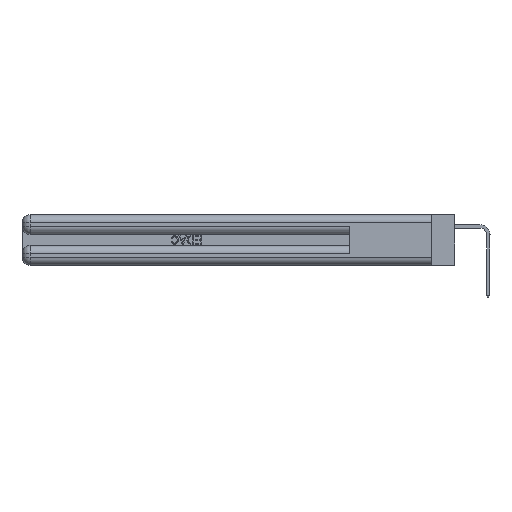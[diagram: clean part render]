
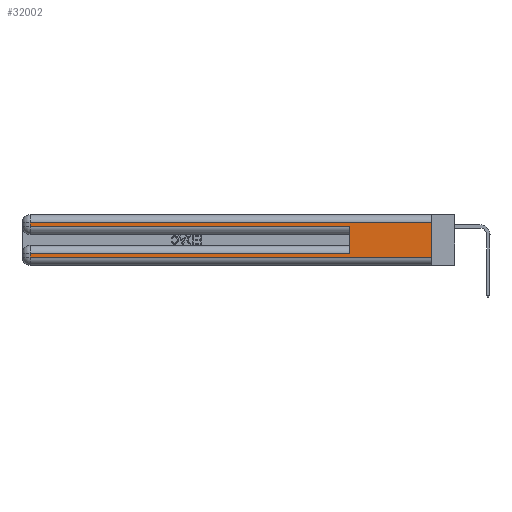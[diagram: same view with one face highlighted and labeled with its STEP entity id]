
A CAD part, left-side view. The second image highlights one B-rep face of the part: STEP entity #32002.
In plain terms, the highlighted planar face has unit normal (-1, 0, 0).
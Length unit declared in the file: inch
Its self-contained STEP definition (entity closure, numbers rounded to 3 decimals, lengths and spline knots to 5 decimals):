
#416 = CARTESIAN_POINT ( 'NONE',  ( 0., 2.94, 0.285 ) ) ;
#809 = VERTEX_POINT ( 'NONE', #416 ) ;
#941 = LINE ( 'NONE', #19264, #25725 ) ;
#985 = EDGE_CURVE ( 'NONE', #2743, #10307, #14815, .T. ) ;
#2058 = DIRECTION ( 'NONE',  ( 0., 0., -1. ) ) ;
#2743 = VERTEX_POINT ( 'NONE', #41487 ) ;
#3011 = VECTOR ( 'NONE', #13478, 39.37008 ) ;
#3036 = CARTESIAN_POINT ( 'NONE',  ( 0., 2.94, 0.31 ) ) ;
#3138 = DIRECTION ( 'NONE',  ( 0., 0., -1. ) ) ;
#3290 = FACE_OUTER_BOUND ( 'NONE', #34576, .T. ) ;
#3439 = CARTESIAN_POINT ( 'NONE',  ( 0., 0., 0.285 ) ) ;
#3688 = VERTEX_POINT ( 'NONE', #37135 ) ;
#4161 = VERTEX_POINT ( 'NONE', #39572 ) ;
#4561 = VERTEX_POINT ( 'NONE', #3036 ) ;
#6394 = DIRECTION ( 'NONE',  ( 0., 1., 0. ) ) ;
#6622 = LINE ( 'NONE', #3439, #31347 ) ;
#8910 = CARTESIAN_POINT ( 'NONE',  ( 0., 2.94, 0.37 ) ) ;
#9658 = LINE ( 'NONE', #32082, #36260 ) ;
#9823 = ORIENTED_EDGE ( 'NONE', *, *, #39728, .F. ) ;
#10307 = VERTEX_POINT ( 'NONE', #21825 ) ;
#10595 = VECTOR ( 'NONE', #39861, 39.37008 ) ;
#11454 = DIRECTION ( 'NONE',  ( 0., 0., 1. ) ) ;
#11680 = LINE ( 'NONE', #13610, #3011 ) ;
#13478 = DIRECTION ( 'NONE',  ( 0., -1., 0. ) ) ;
#13610 = CARTESIAN_POINT ( 'NONE',  ( 0., 0., 0.06 ) ) ;
#14056 = EDGE_CURVE ( 'NONE', #809, #10307, #6622, .T. ) ;
#14815 = LINE ( 'NONE', #27477, #23343 ) ;
#14848 = LINE ( 'NONE', #33110, #22363 ) ;
#14862 = EDGE_CURVE ( 'NONE', #4161, #3688, #11680, .T. ) ;
#16480 = ORIENTED_EDGE ( 'NONE', *, *, #25619, .T. ) ;
#17704 = CARTESIAN_POINT ( 'NONE',  ( 0., 0., 0.31 ) ) ;
#17847 = CARTESIAN_POINT ( 'NONE',  ( 0., 2.94, 0.085 ) ) ;
#19086 = LINE ( 'NONE', #8910, #35114 ) ;
#19155 = LINE ( 'NONE', #27089, #10595 ) ;
#19264 = CARTESIAN_POINT ( 'NONE',  ( 0., 2.94, 0.37 ) ) ;
#21438 = DIRECTION ( 'NONE',  ( 1., 0., 0. ) ) ;
#21825 = CARTESIAN_POINT ( 'NONE',  ( 0., 0.6, 0.285 ) ) ;
#22363 = VECTOR ( 'NONE', #26653, 39.37008 ) ;
#23233 = VERTEX_POINT ( 'NONE', #17847 ) ;
#23343 = VECTOR ( 'NONE', #11454, 39.37008 ) ;
#24822 = EDGE_CURVE ( 'NONE', #4561, #809, #941, .T. ) ;
#25619 = EDGE_CURVE ( 'NONE', #23233, #4161, #19086, .T. ) ;
#25725 = VECTOR ( 'NONE', #3138, 39.37008 ) ;
#26653 = DIRECTION ( 'NONE',  ( 0., 0., -1. ) ) ;
#26655 = AXIS2_PLACEMENT_3D ( 'NONE', #40238, #21438, #2058 ) ;
#27089 = CARTESIAN_POINT ( 'NONE',  ( 0., 0., 0.085 ) ) ;
#27477 = CARTESIAN_POINT ( 'NONE',  ( 0., 0.6, 0.145 ) ) ;
#29108 = EDGE_CURVE ( 'NONE', #41019, #4561, #9658, .T. ) ;
#29252 = DIRECTION ( 'NONE',  ( 0., -1., 0. ) ) ;
#29908 = EDGE_CURVE ( 'NONE', #2743, #23233, #19155, .T. ) ;
#31347 = VECTOR ( 'NONE', #29252, 39.37008 ) ;
#31430 = DIRECTION ( 'NONE',  ( 0., 0., -1. ) ) ;
#31756 = ORIENTED_EDGE ( 'NONE', *, *, #14056, .T. ) ;
#32002 = ADVANCED_FACE ( 'NONE', ( #3290 ), #40512, .F. ) ;
#32082 = CARTESIAN_POINT ( 'NONE',  ( 0., 0., 0.31 ) ) ;
#32940 = ORIENTED_EDGE ( 'NONE', *, *, #985, .F. ) ;
#33110 = CARTESIAN_POINT ( 'NONE',  ( 0., 0., 0.37 ) ) ;
#34576 = EDGE_LOOP ( 'NONE', ( #9823, #37883, #37714, #31756, #32940, #37865, #16480, #35049 ) ) ;
#35049 = ORIENTED_EDGE ( 'NONE', *, *, #14862, .T. ) ;
#35114 = VECTOR ( 'NONE', #31430, 39.37008 ) ;
#36260 = VECTOR ( 'NONE', #6394, 39.37008 ) ;
#37135 = CARTESIAN_POINT ( 'NONE',  ( 0., 0., 0.06 ) ) ;
#37714 = ORIENTED_EDGE ( 'NONE', *, *, #24822, .T. ) ;
#37865 = ORIENTED_EDGE ( 'NONE', *, *, #29908, .T. ) ;
#37883 = ORIENTED_EDGE ( 'NONE', *, *, #29108, .T. ) ;
#39572 = CARTESIAN_POINT ( 'NONE',  ( 0., 2.94, 0.06 ) ) ;
#39728 = EDGE_CURVE ( 'NONE', #41019, #3688, #14848, .T. ) ;
#39861 = DIRECTION ( 'NONE',  ( 0., 1., 0. ) ) ;
#40238 = CARTESIAN_POINT ( 'NONE',  ( 0., 0., 0.37 ) ) ;
#40512 = PLANE ( 'NONE',  #26655 ) ;
#41019 = VERTEX_POINT ( 'NONE', #17704 ) ;
#41487 = CARTESIAN_POINT ( 'NONE',  ( 0., 0.6, 0.085 ) ) ;
